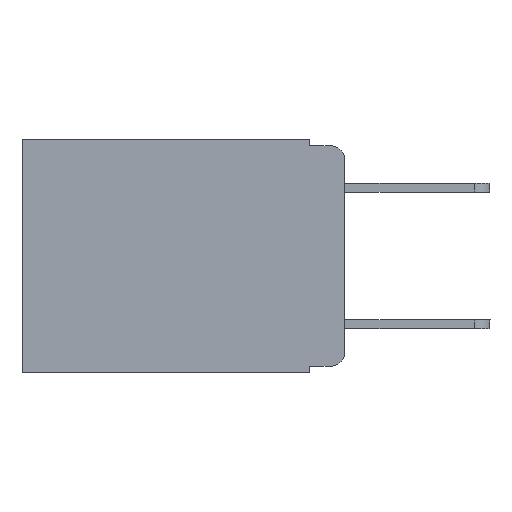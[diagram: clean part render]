
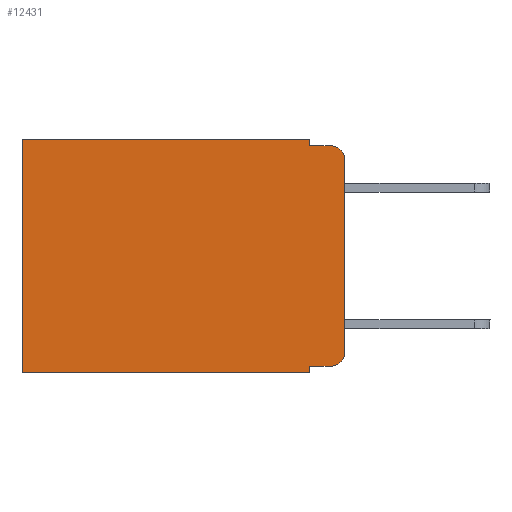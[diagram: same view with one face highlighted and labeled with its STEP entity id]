
A CAD part, left-side view. The second image highlights one B-rep face of the part: STEP entity #12431.
In plain terms, the highlighted planar face has unit normal (-1, 0, 0).
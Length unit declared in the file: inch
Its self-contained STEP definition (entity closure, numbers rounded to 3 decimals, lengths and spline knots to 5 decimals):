
#27 = LINE ( 'NONE', #11619, #3552 ) ;
#47 = CARTESIAN_POINT ( 'NONE',  ( 0.298, 0., 0. ) ) ;
#84 = CARTESIAN_POINT ( 'NONE',  ( 0.298, 0., -0.03 ) ) ;
#146 = EDGE_CURVE ( 'NONE', #15389, #15170, #697, .T. ) ;
#228 = VERTEX_POINT ( 'NONE', #12022 ) ;
#484 = LINE ( 'NONE', #47, #5743 ) ;
#486 = ORIENTED_EDGE ( 'NONE', *, *, #9553, .F. ) ;
#546 = LINE ( 'NONE', #7619, #13143 ) ;
#682 = CARTESIAN_POINT ( 'NONE',  ( 0.298, 0., -0.313 ) ) ;
#697 = LINE ( 'NONE', #2308, #2909 ) ;
#824 = EDGE_CURVE ( 'NONE', #3430, #9838, #484, .T. ) ;
#948 = CARTESIAN_POINT ( 'NONE',  ( 0.298, 0.473, -0.343 ) ) ;
#1314 = VERTEX_POINT ( 'NONE', #1593 ) ;
#1521 = VERTEX_POINT ( 'NONE', #9117 ) ;
#1593 = CARTESIAN_POINT ( 'NONE',  ( 0.298, 0.02, -0.333 ) ) ;
#1698 = ORIENTED_EDGE ( 'NONE', *, *, #6931, .T. ) ;
#1794 = CARTESIAN_POINT ( 'NONE',  ( 0.298, 0.051, -0.333 ) ) ;
#1944 = CARTESIAN_POINT ( 'NONE',  ( 0.298, 0.473, 0. ) ) ;
#2213 = ORIENTED_EDGE ( 'NONE', *, *, #3852, .T. ) ;
#2265 = DIRECTION ( 'NONE',  ( 0., 0., -1. ) ) ;
#2308 = CARTESIAN_POINT ( 'NONE',  ( 0.298, 0., -0.343 ) ) ;
#2546 = CARTESIAN_POINT ( 'NONE',  ( 0.298, 0.051, -0.343 ) ) ;
#2704 = CARTESIAN_POINT ( 'NONE',  ( 0.298, 0.051, -0.01 ) ) ;
#2813 = EDGE_CURVE ( 'NONE', #4627, #15170, #2850, .T. ) ;
#2850 = LINE ( 'NONE', #1944, #13063 ) ;
#2909 = VECTOR ( 'NONE', #7329, 39.37008 ) ;
#2926 = DIRECTION ( 'NONE',  ( 0., 0., -1. ) ) ;
#3029 = EDGE_CURVE ( 'NONE', #3430, #228, #15133, .T. ) ;
#3430 = VERTEX_POINT ( 'NONE', #84 ) ;
#3432 = CARTESIAN_POINT ( 'NONE',  ( 0.298, 0.473, 0. ) ) ;
#3552 = VECTOR ( 'NONE', #10344, 39.37008 ) ;
#3652 = DIRECTION ( 'NONE',  ( 0., 0., -1. ) ) ;
#3852 = EDGE_CURVE ( 'NONE', #8240, #4627, #27, .T. ) ;
#3961 = AXIS2_PLACEMENT_3D ( 'NONE', #8481, #14484, #3652 ) ;
#4010 = DIRECTION ( 'NONE',  ( 0., -1., 0. ) ) ;
#4623 = EDGE_LOOP ( 'NONE', ( #11404, #13851, #486, #14647, #2213, #4652, #8183, #6045, #10953, #1698 ) ) ;
#4627 = VERTEX_POINT ( 'NONE', #3432 ) ;
#4652 = ORIENTED_EDGE ( 'NONE', *, *, #2813, .T. ) ;
#4746 = FACE_OUTER_BOUND ( 'NONE', #4623, .T. ) ;
#5104 = DIRECTION ( 'NONE',  ( 0., -1., 0. ) ) ;
#5354 = LINE ( 'NONE', #15460, #12935 ) ;
#5514 = CARTESIAN_POINT ( 'NONE',  ( 0.298, 0.02, -0.313 ) ) ;
#5694 = EDGE_CURVE ( 'NONE', #12574, #1314, #546, .T. ) ;
#5743 = VECTOR ( 'NONE', #6842, 39.37008 ) ;
#6045 = ORIENTED_EDGE ( 'NONE', *, *, #7389, .F. ) ;
#6695 = VECTOR ( 'NONE', #4010, 39.37008 ) ;
#6842 = DIRECTION ( 'NONE',  ( 0., 0., -1. ) ) ;
#6931 = EDGE_CURVE ( 'NONE', #1314, #9838, #7533, .T. ) ;
#7329 = DIRECTION ( 'NONE',  ( 0., 1., 0. ) ) ;
#7363 = CARTESIAN_POINT ( 'NONE',  ( 0.298, 0., 0. ) ) ;
#7389 = EDGE_CURVE ( 'NONE', #12574, #15389, #15248, .T. ) ;
#7533 = CIRCLE ( 'NONE', #8391, 0.02 ) ;
#7619 = CARTESIAN_POINT ( 'NONE',  ( 0.298, 0.051, -0.333 ) ) ;
#7766 = CARTESIAN_POINT ( 'NONE',  ( 0.298, 0.051, 0. ) ) ;
#8183 = ORIENTED_EDGE ( 'NONE', *, *, #146, .F. ) ;
#8240 = VERTEX_POINT ( 'NONE', #14467 ) ;
#8391 = AXIS2_PLACEMENT_3D ( 'NONE', #5514, #15180, #2926 ) ;
#8481 = CARTESIAN_POINT ( 'NONE',  ( 0.298, 0.02, -0.03 ) ) ;
#8830 = VECTOR ( 'NONE', #13872, 39.37008 ) ;
#9117 = CARTESIAN_POINT ( 'NONE',  ( 0.298, 0.051, -0.01 ) ) ;
#9518 = DIRECTION ( 'NONE',  ( 1., 0., 0. ) ) ;
#9553 = EDGE_CURVE ( 'NONE', #1521, #228, #9890, .T. ) ;
#9838 = VERTEX_POINT ( 'NONE', #682 ) ;
#9890 = LINE ( 'NONE', #2704, #6695 ) ;
#10344 = DIRECTION ( 'NONE',  ( 0., 1., 0. ) ) ;
#10407 = DIRECTION ( 'NONE',  ( 0., 0., -1. ) ) ;
#10769 = DIRECTION ( 'NONE',  ( 0., 0., -1. ) ) ;
#10953 = ORIENTED_EDGE ( 'NONE', *, *, #5694, .T. ) ;
#11404 = ORIENTED_EDGE ( 'NONE', *, *, #824, .F. ) ;
#11619 = CARTESIAN_POINT ( 'NONE',  ( 0.298, 0., 0. ) ) ;
#12022 = CARTESIAN_POINT ( 'NONE',  ( 0.298, 0.02, -0.01 ) ) ;
#12431 = ADVANCED_FACE ( 'NONE', ( #4746 ), #14554, .F. ) ;
#12574 = VERTEX_POINT ( 'NONE', #1794 ) ;
#12882 = EDGE_CURVE ( 'NONE', #8240, #1521, #5354, .T. ) ;
#12935 = VECTOR ( 'NONE', #10769, 39.37008 ) ;
#13063 = VECTOR ( 'NONE', #10407, 39.37008 ) ;
#13143 = VECTOR ( 'NONE', #5104, 39.37008 ) ;
#13259 = AXIS2_PLACEMENT_3D ( 'NONE', #7363, #9518, #2265 ) ;
#13851 = ORIENTED_EDGE ( 'NONE', *, *, #3029, .T. ) ;
#13872 = DIRECTION ( 'NONE',  ( 0., 0., -1. ) ) ;
#14467 = CARTESIAN_POINT ( 'NONE',  ( 0.298, 0.051, 0. ) ) ;
#14484 = DIRECTION ( 'NONE',  ( -1., 0., 0. ) ) ;
#14554 = PLANE ( 'NONE',  #13259 ) ;
#14647 = ORIENTED_EDGE ( 'NONE', *, *, #12882, .F. ) ;
#15133 = CIRCLE ( 'NONE', #3961, 0.02 ) ;
#15170 = VERTEX_POINT ( 'NONE', #948 ) ;
#15180 = DIRECTION ( 'NONE',  ( -1., 0., 0. ) ) ;
#15248 = LINE ( 'NONE', #7766, #8830 ) ;
#15389 = VERTEX_POINT ( 'NONE', #2546 ) ;
#15460 = CARTESIAN_POINT ( 'NONE',  ( 0.298, 0.051, 0. ) ) ;
